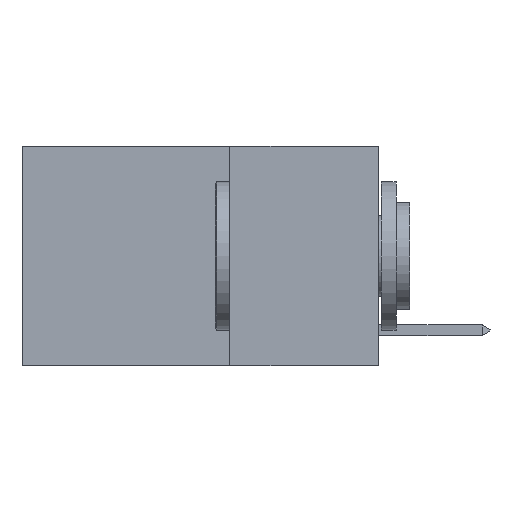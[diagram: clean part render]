
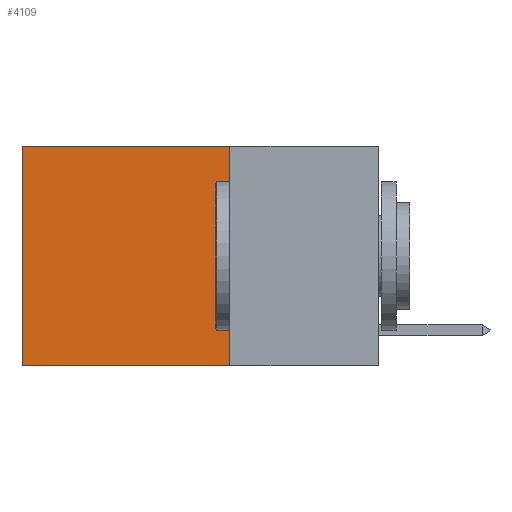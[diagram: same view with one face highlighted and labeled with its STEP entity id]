
A CAD part, left-side view. The second image highlights one B-rep face of the part: STEP entity #4109.
In plain terms, the highlighted planar face has unit normal (-1, 0, 0).
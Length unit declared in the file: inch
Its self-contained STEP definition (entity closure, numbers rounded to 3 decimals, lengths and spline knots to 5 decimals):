
#169 = EDGE_CURVE ( 'NONE', #1912, #8022, #3242, .T. ) ;
#390 = CARTESIAN_POINT ( 'NONE',  ( 0.2625, 0.25, 0. ) ) ;
#1750 = ORIENTED_EDGE ( 'NONE', *, *, #12502, .F. ) ;
#1751 = VECTOR ( 'NONE', #9969, 39.37008 ) ;
#1912 = VERTEX_POINT ( 'NONE', #7784 ) ;
#2136 = EDGE_CURVE ( 'NONE', #1912, #4450, #7347, .T. ) ;
#2435 = EDGE_LOOP ( 'NONE', ( #3190, #1750, #4054, #4533 ) ) ;
#2788 = VERTEX_POINT ( 'NONE', #12064 ) ;
#3071 = CARTESIAN_POINT ( 'NONE',  ( 0.2625, 0.25, 0. ) ) ;
#3190 = ORIENTED_EDGE ( 'NONE', *, *, #11936, .T. ) ;
#3192 = LINE ( 'NONE', #4947, #7050 ) ;
#3242 = LINE ( 'NONE', #390, #5545 ) ;
#4054 = ORIENTED_EDGE ( 'NONE', *, *, #2136, .F. ) ;
#4109 = ADVANCED_FACE ( 'NONE', ( #5141 ), #9587, .F. ) ;
#4450 = VERTEX_POINT ( 'NONE', #4816 ) ;
#4533 = ORIENTED_EDGE ( 'NONE', *, *, #169, .T. ) ;
#4816 = CARTESIAN_POINT ( 'NONE',  ( 0.2625, 0.25, -0.37 ) ) ;
#4947 = CARTESIAN_POINT ( 'NONE',  ( 0.2625, 0.6, 0. ) ) ;
#5141 = FACE_OUTER_BOUND ( 'NONE', #2435, .T. ) ;
#5545 = VECTOR ( 'NONE', #12159, 39.37008 ) ;
#5729 = DIRECTION ( 'NONE',  ( 0., 1., 0. ) ) ;
#5765 = CARTESIAN_POINT ( 'NONE',  ( 0.2625, 0.6, 0. ) ) ;
#6189 = AXIS2_PLACEMENT_3D ( 'NONE', #10510, #6675, #7813 ) ;
#6675 = DIRECTION ( 'NONE',  ( 1., 0., 0. ) ) ;
#7050 = VECTOR ( 'NONE', #11030, 39.37008 ) ;
#7347 = LINE ( 'NONE', #3071, #1751 ) ;
#7784 = CARTESIAN_POINT ( 'NONE',  ( 0.2625, 0.25, 0. ) ) ;
#7813 = DIRECTION ( 'NONE',  ( 0., 0., -1. ) ) ;
#8022 = VERTEX_POINT ( 'NONE', #5765 ) ;
#8888 = LINE ( 'NONE', #10525, #12077 ) ;
#9587 = PLANE ( 'NONE',  #6189 ) ;
#9969 = DIRECTION ( 'NONE',  ( 0., 0., -1. ) ) ;
#10510 = CARTESIAN_POINT ( 'NONE',  ( 0.2625, 0.25, 0. ) ) ;
#10525 = CARTESIAN_POINT ( 'NONE',  ( 0.2625, 0.25, -0.37 ) ) ;
#11030 = DIRECTION ( 'NONE',  ( 0., 0., -1. ) ) ;
#11936 = EDGE_CURVE ( 'NONE', #8022, #2788, #3192, .T. ) ;
#12064 = CARTESIAN_POINT ( 'NONE',  ( 0.2625, 0.6, -0.37 ) ) ;
#12077 = VECTOR ( 'NONE', #5729, 39.37008 ) ;
#12159 = DIRECTION ( 'NONE',  ( 0., 1., 0. ) ) ;
#12502 = EDGE_CURVE ( 'NONE', #4450, #2788, #8888, .T. ) ;
